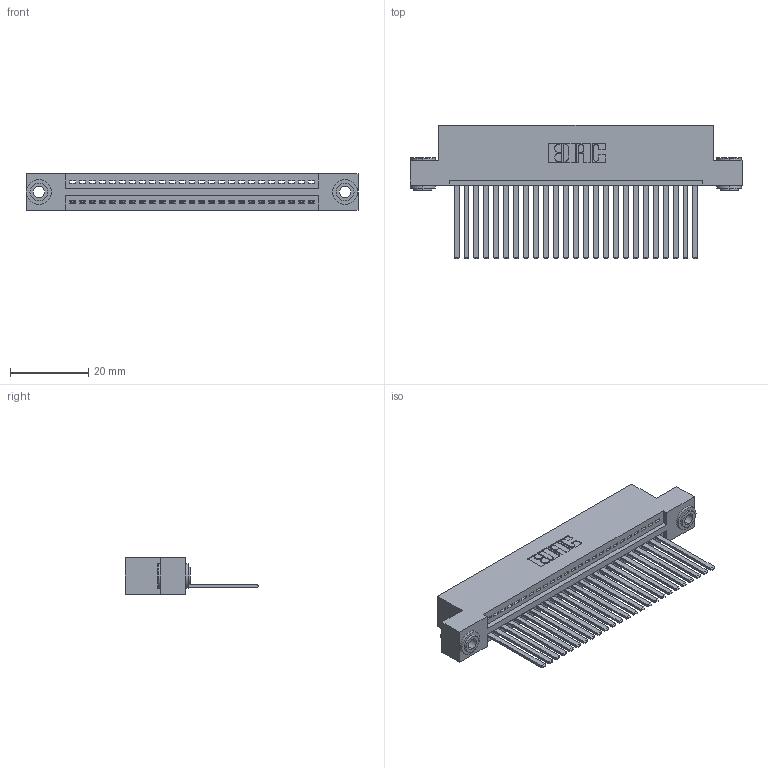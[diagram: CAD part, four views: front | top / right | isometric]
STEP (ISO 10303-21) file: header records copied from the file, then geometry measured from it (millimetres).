
FILE_DESCRIPTION (( 'STEP AP203' ), '1' );
FILE_NAME ('395-025-544-103.STEP', '2018-11-09T13:20:26', ( '' ), ( '' ), 'SwSTEP 2.0', 'SolidWorks 2016', '' );
FILE_SCHEMA (( 'CONFIG_CONTROL_DESIGN' ));
Length unit declared in the file: inch
Products named in the file (4): 395-025-544-103; 345 Part_Flush Mounting Lugs - 0.156 Dia-TH; 345-250-002_345-250-002-102; 345-292-001_345-293-144
Assembly tree (28 placements, depth 2):
  395-025-544-103
    345 Part_Flush Mounting Lugs - 0.156 Dia-TH
    345-292-001_345-293-144  x25
    345-250-002_345-250-002-102  x2
Bounding box: 84.71 x 33.96 x 9.4 mm (x, y, z)
Volume: 8215.4 mm3; surface area: 11770.2 mm2
Topology: 28 solids, 28 shells, 1464 faces, 4367 edges, 2874 vertices
Faces by surface type: plane 990, cylinder 466, cone 8
Entity records: 21570 total; most frequent: CARTESIAN_POINT 3714, ORIENTED_EDGE 3666, DIRECTION 3297, EDGE_CURVE 1833, LINE 1581, VECTOR 1581, VERTEX_POINT 1218, AXIS2_PLACEMENT_3D 858
